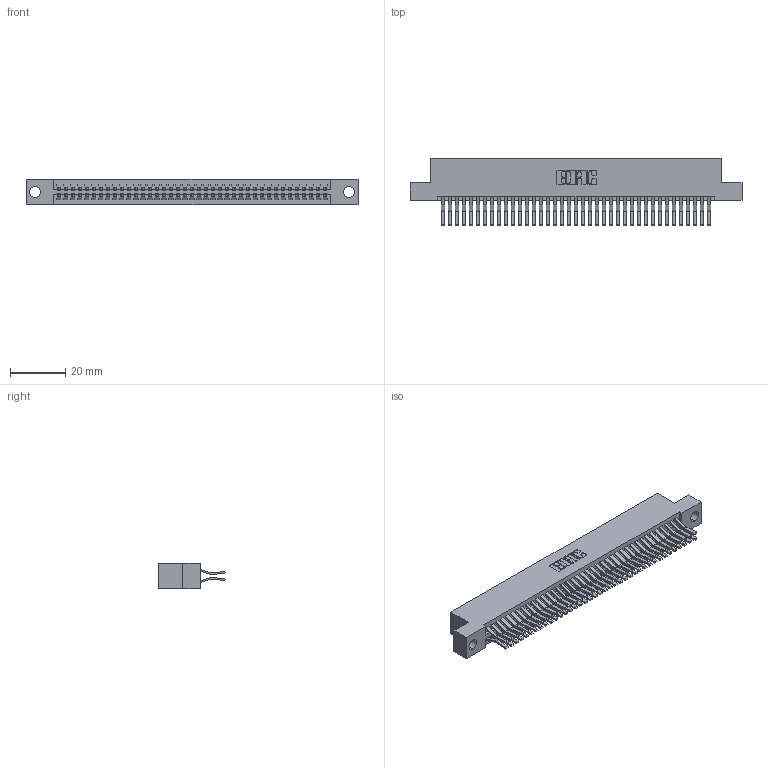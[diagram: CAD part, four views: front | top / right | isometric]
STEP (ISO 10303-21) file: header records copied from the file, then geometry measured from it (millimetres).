
FILE_DESCRIPTION (( 'STEP AP203' ), '1' );
FILE_NAME ('395-078-560-204.STEP', '2018-11-28T02:23:34', ( '' ), ( '' ), 'SwSTEP 2.0', 'SolidWorks 2016', '' );
FILE_SCHEMA (( 'CONFIG_CONTROL_DESIGN' ));
Length unit declared in the file: inch
Products named in the file (3): 345 Part_Flush Mounting Lugs - 0.156 Dia-TH; 395-078-560-204; 345-292-001_560 Tail
Assembly tree (79 placements, depth 2):
  395-078-560-204
    345 Part_Flush Mounting Lugs - 0.156 Dia-TH
    345-292-001_560 Tail  x78
Bounding box: 120.27 x 24.45 x 9.4 mm (x, y, z)
Volume: 12078.6 mm3; surface area: 18926.2 mm2
Topology: 79 solids, 79 shells, 4182 faces, 12431 edges, 8182 vertices
Faces by surface type: plane 2654, cylinder 1528
Entity records: 31095 total; most frequent: CARTESIAN_POINT 5216, ORIENTED_EDGE 5150, DIRECTION 4607, EDGE_CURVE 2575, LINE 2283, VECTOR 2283, VERTEX_POINT 1714, AXIS2_PLACEMENT_3D 1162
